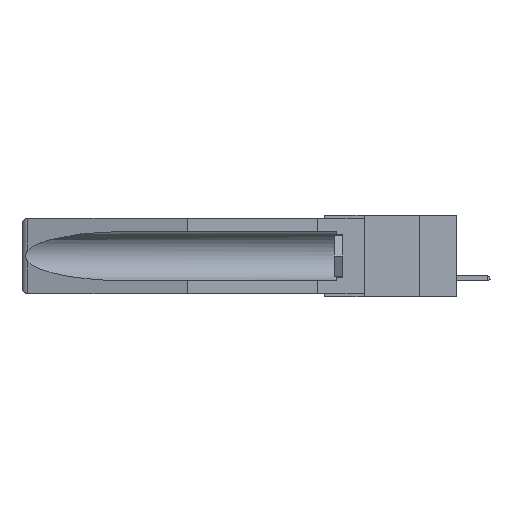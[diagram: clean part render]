
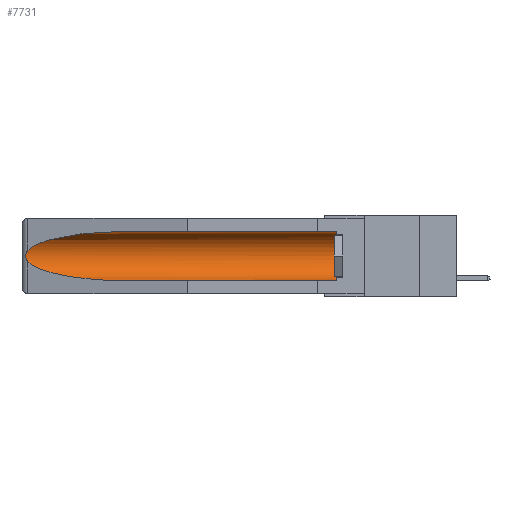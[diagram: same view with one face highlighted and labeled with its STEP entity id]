
A CAD part, left-side view. The second image highlights one B-rep face of the part: STEP entity #7731.
In plain terms, the highlighted cylindrical face has radius 2.857 mm (diameter 5.715 mm), a partial arc.
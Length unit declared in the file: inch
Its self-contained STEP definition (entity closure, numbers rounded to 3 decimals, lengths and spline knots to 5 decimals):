
#487 = DIRECTION ( 'NONE',  ( 0., 1., 0. ) ) ;
#552 = DIRECTION ( 'NONE',  ( 0., 1., 0. ) ) ;
#714 = EDGE_CURVE ( 'NONE', #1566, #13793, #11455, .T. ) ;
#892 = EDGE_LOOP ( 'NONE', ( #1555, #9413, #1376, #8698, #6274, #18736 ) ) ;
#1103 = DIRECTION ( 'NONE',  ( 0., 1., 0. ) ) ;
#1376 = ORIENTED_EDGE ( 'NONE', *, *, #18421, .T. ) ;
#1552 = CARTESIAN_POINT ( 'NONE',  ( 0.2673, 1.5327, -0.16383 ) ) ;
#1555 = ORIENTED_EDGE ( 'NONE', *, *, #18923, .T. ) ;
#1566 = VERTEX_POINT ( 'NONE', #4344 ) ;
#2659 = CYLINDRICAL_SURFACE ( 'NONE', #12485, 0.1125 ) ;
#2666 = CARTESIAN_POINT ( 'NONE',  ( 0.26537, 1.52718, -0.14972 ) ) ;
#3029 = CARTESIAN_POINT ( 'NONE',  ( 0.2675, 1.53308, -0.17534 ) ) ;
#3694 = B_SPLINE_CURVE_WITH_KNOTS ( 'NONE', 3,
 ( #7469, #4715, #11964, #1552, #11850, #3029, #13331, #17825, #14886, #6043 ),
 .UNSPECIFIED., .F., .F.,
 ( 4, 2, 2, 2, 4 ),
 ( 0., 0.00029, 0.00058, 0.00087, 0.00117 ),
 .UNSPECIFIED. ) ;
#4013 = CARTESIAN_POINT ( 'NONE',  ( 0.155, 0.126, -0.1715 ) ) ;
#4344 = CARTESIAN_POINT ( 'NONE',  ( 0.155, 0.126, -0.284 ) ) ;
#4398 = EDGE_CURVE ( 'NONE', #13793, #7771, #9378, .T. ) ;
#4715 = CARTESIAN_POINT ( 'NONE',  ( 0.26597, 1.52961, -0.15275 ) ) ;
#4967 = VECTOR ( 'NONE', #1103, 39.37008 ) ;
#5248 = CARTESIAN_POINT ( 'NONE',  ( 0.26537, 1.52718, -0.14972 ) ) ;
#5609 = CARTESIAN_POINT ( 'NONE',  ( 0.155, 1.07973, -0.059 ) ) ;
#6043 = CARTESIAN_POINT ( 'NONE',  ( 0.26537, 1.52718, -0.19328 ) ) ;
#6274 = ORIENTED_EDGE ( 'NONE', *, *, #714, .T. ) ;
#6304 =( BOUNDED_CURVE ( )  B_SPLINE_CURVE ( 3, ( #5609, #13074, #9988, #2666 ),
 .UNSPECIFIED., .F., .F. ) 
 B_SPLINE_CURVE_WITH_KNOTS ( ( 4, 4 ),
 ( 4.71239, 6.08839 ),
 .UNSPECIFIED. ) 
 CURVE ( )  GEOMETRIC_REPRESENTATION_ITEM ( )  RATIONAL_B_SPLINE_CURVE ( ( 1., 0.848, 0.848, 1. ) ) 
 REPRESENTATION_ITEM ( '' )  );
#6413 = VERTEX_POINT ( 'NONE', #18014 ) ;
#6512 = CARTESIAN_POINT ( 'NONE',  ( 0.155, 1.07973, -0.284 ) ) ;
#7004 = EDGE_CURVE ( 'NONE', #1566, #6413, #7929, .T. ) ;
#7378 = CARTESIAN_POINT ( 'NONE',  ( 0.155, 0.126, -0.059 ) ) ;
#7431 = AXIS2_PLACEMENT_3D ( 'NONE', #4013, #17133, #8386 ) ;
#7469 = CARTESIAN_POINT ( 'NONE',  ( 0.26537, 1.52718, -0.14972 ) ) ;
#7485 = VECTOR ( 'NONE', #552, 39.37008 ) ;
#7731 = ADVANCED_FACE ( 'NONE', ( #17436 ), #2659, .F. ) ;
#7771 = VERTEX_POINT ( 'NONE', #16994 ) ;
#7929 = LINE ( 'NONE', #12180, #7485 ) ;
#8386 = DIRECTION ( 'NONE',  ( 0., 0., 1. ) ) ;
#8670 =( BOUNDED_CURVE ( )  B_SPLINE_CURVE ( 3, ( #16930, #12366, #9579, #6512 ),
 .UNSPECIFIED., .F., .F. ) 
 B_SPLINE_CURVE_WITH_KNOTS ( ( 4, 4 ),
 ( 0.1948, 1.5708 ),
 .UNSPECIFIED. ) 
 CURVE ( )  GEOMETRIC_REPRESENTATION_ITEM ( )  RATIONAL_B_SPLINE_CURVE ( ( 1., 0.848, 0.848, 1. ) ) 
 REPRESENTATION_ITEM ( '' )  );
#8698 = ORIENTED_EDGE ( 'NONE', *, *, #7004, .F. ) ;
#9159 = DIRECTION ( 'NONE',  ( 0., 0., 1. ) ) ;
#9378 = LINE ( 'NONE', #17220, #4967 ) ;
#9413 = ORIENTED_EDGE ( 'NONE', *, *, #13060, .T. ) ;
#9579 = CARTESIAN_POINT ( 'NONE',  ( 0.21114, 1.30732, -0.284 ) ) ;
#9988 = CARTESIAN_POINT ( 'NONE',  ( 0.25451, 1.48313, -0.09465 ) ) ;
#11455 = CIRCLE ( 'NONE', #7431, 0.1125 ) ;
#11850 = CARTESIAN_POINT ( 'NONE',  ( 0.2675, 1.53308, -0.16763 ) ) ;
#11964 = CARTESIAN_POINT ( 'NONE',  ( 0.26654, 1.53092, -0.15636 ) ) ;
#12180 = CARTESIAN_POINT ( 'NONE',  ( 0.155, -0.30754, -0.284 ) ) ;
#12366 = CARTESIAN_POINT ( 'NONE',  ( 0.25451, 1.48313, -0.24835 ) ) ;
#12485 = AXIS2_PLACEMENT_3D ( 'NONE', #16605, #487, #9159 ) ;
#13060 = EDGE_CURVE ( 'NONE', #15654, #17875, #3694, .T. ) ;
#13074 = CARTESIAN_POINT ( 'NONE',  ( 0.21114, 1.30732, -0.059 ) ) ;
#13331 = CARTESIAN_POINT ( 'NONE',  ( 0.2673, 1.53269, -0.17917 ) ) ;
#13793 = VERTEX_POINT ( 'NONE', #7378 ) ;
#14886 = CARTESIAN_POINT ( 'NONE',  ( 0.26597, 1.5296, -0.19026 ) ) ;
#15654 = VERTEX_POINT ( 'NONE', #5248 ) ;
#16605 = CARTESIAN_POINT ( 'NONE',  ( 0.155, -0.30754, -0.1715 ) ) ;
#16930 = CARTESIAN_POINT ( 'NONE',  ( 0.26537, 1.52718, -0.19328 ) ) ;
#16994 = CARTESIAN_POINT ( 'NONE',  ( 0.155, 1.07973, -0.059 ) ) ;
#17133 = DIRECTION ( 'NONE',  ( 0., -1., 0. ) ) ;
#17220 = CARTESIAN_POINT ( 'NONE',  ( 0.155, -0.30754, -0.059 ) ) ;
#17436 = FACE_OUTER_BOUND ( 'NONE', #892, .T. ) ;
#17825 = CARTESIAN_POINT ( 'NONE',  ( 0.26655, 1.53094, -0.18657 ) ) ;
#17875 = VERTEX_POINT ( 'NONE', #18175 ) ;
#18014 = CARTESIAN_POINT ( 'NONE',  ( 0.155, 1.07973, -0.284 ) ) ;
#18175 = CARTESIAN_POINT ( 'NONE',  ( 0.26537, 1.52718, -0.19328 ) ) ;
#18421 = EDGE_CURVE ( 'NONE', #17875, #6413, #8670, .T. ) ;
#18736 = ORIENTED_EDGE ( 'NONE', *, *, #4398, .T. ) ;
#18923 = EDGE_CURVE ( 'NONE', #7771, #15654, #6304, .T. ) ;
